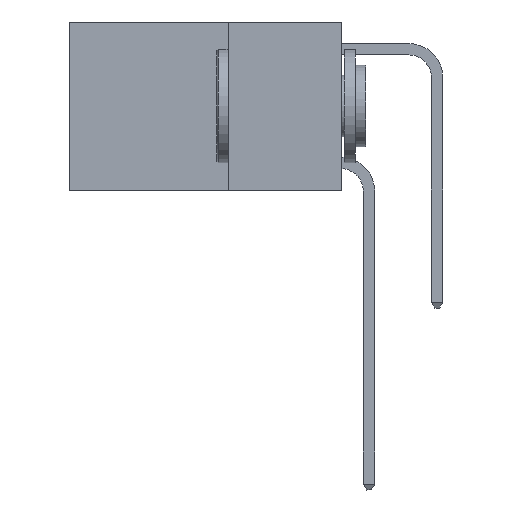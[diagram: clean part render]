
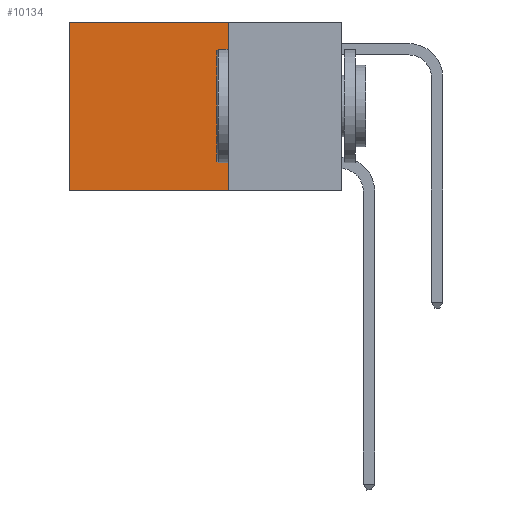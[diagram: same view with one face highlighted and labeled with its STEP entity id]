
A CAD part, left-side view. The second image highlights one B-rep face of the part: STEP entity #10134.
In plain terms, the highlighted planar face has unit normal (-1, 0, 0).
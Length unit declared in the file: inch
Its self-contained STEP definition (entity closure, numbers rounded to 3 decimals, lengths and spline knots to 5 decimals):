
#15 = CARTESIAN_POINT ( 'NONE',  ( 0.2625, 0.25, 0. ) ) ;
#189 = EDGE_CURVE ( 'NONE', #3305, #6437, #2863, .T. ) ;
#679 = VECTOR ( 'NONE', #2874, 39.37008 ) ;
#877 = DIRECTION ( 'NONE',  ( 0., 0., -1. ) ) ;
#940 = DIRECTION ( 'NONE',  ( 1., 0., 0. ) ) ;
#962 = LINE ( 'NONE', #8248, #679 ) ;
#1781 = AXIS2_PLACEMENT_3D ( 'NONE', #15, #940, #7257 ) ;
#1857 = LINE ( 'NONE', #5341, #11056 ) ;
#2577 = ORIENTED_EDGE ( 'NONE', *, *, #189, .T. ) ;
#2863 = LINE ( 'NONE', #5335, #9460 ) ;
#2874 = DIRECTION ( 'NONE',  ( 0., 0., -1. ) ) ;
#3305 = VERTEX_POINT ( 'NONE', #5887 ) ;
#4360 = EDGE_LOOP ( 'NONE', ( #11431, #6763, #9263, #2577 ) ) ;
#5335 = CARTESIAN_POINT ( 'NONE',  ( 0.2625, 0.25, 0. ) ) ;
#5341 = CARTESIAN_POINT ( 'NONE',  ( 0.2625, 0.25, -0.37 ) ) ;
#5460 = PLANE ( 'NONE',  #1781 ) ;
#5615 = VERTEX_POINT ( 'NONE', #9468 ) ;
#5887 = CARTESIAN_POINT ( 'NONE',  ( 0.2625, 0.25, 0. ) ) ;
#5910 = VECTOR ( 'NONE', #877, 39.37008 ) ;
#6363 = EDGE_CURVE ( 'NONE', #7246, #5615, #1857, .T. ) ;
#6437 = VERTEX_POINT ( 'NONE', #7244 ) ;
#6763 = ORIENTED_EDGE ( 'NONE', *, *, #6363, .F. ) ;
#7193 = CARTESIAN_POINT ( 'NONE',  ( 0.2625, 0.6, 0. ) ) ;
#7244 = CARTESIAN_POINT ( 'NONE',  ( 0.2625, 0.6, 0. ) ) ;
#7246 = VERTEX_POINT ( 'NONE', #8477 ) ;
#7257 = DIRECTION ( 'NONE',  ( 0., 0., -1. ) ) ;
#7260 = FACE_OUTER_BOUND ( 'NONE', #4360, .T. ) ;
#7673 = EDGE_CURVE ( 'NONE', #3305, #7246, #962, .T. ) ;
#7703 = LINE ( 'NONE', #7193, #5910 ) ;
#8120 = DIRECTION ( 'NONE',  ( 0., 1., 0. ) ) ;
#8248 = CARTESIAN_POINT ( 'NONE',  ( 0.2625, 0.25, 0. ) ) ;
#8477 = CARTESIAN_POINT ( 'NONE',  ( 0.2625, 0.25, -0.37 ) ) ;
#8914 = DIRECTION ( 'NONE',  ( 0., 1., 0. ) ) ;
#9263 = ORIENTED_EDGE ( 'NONE', *, *, #7673, .F. ) ;
#9372 = EDGE_CURVE ( 'NONE', #6437, #5615, #7703, .T. ) ;
#9460 = VECTOR ( 'NONE', #8120, 39.37008 ) ;
#9468 = CARTESIAN_POINT ( 'NONE',  ( 0.2625, 0.6, -0.37 ) ) ;
#10134 = ADVANCED_FACE ( 'NONE', ( #7260 ), #5460, .F. ) ;
#11056 = VECTOR ( 'NONE', #8914, 39.37008 ) ;
#11431 = ORIENTED_EDGE ( 'NONE', *, *, #9372, .T. ) ;
